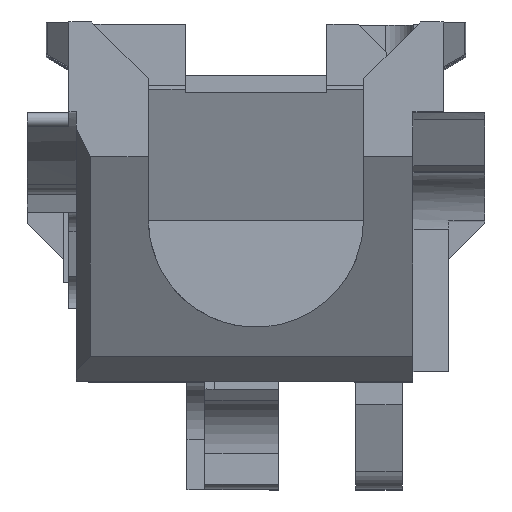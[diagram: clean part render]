
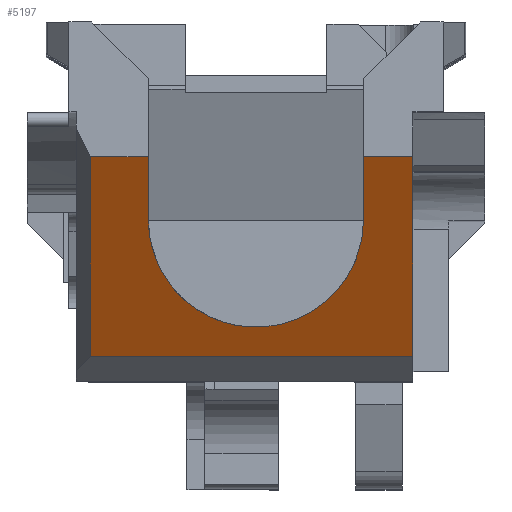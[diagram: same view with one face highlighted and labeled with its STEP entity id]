
A CAD part, top view. The second image highlights one B-rep face of the part: STEP entity #5197.
In plain terms, the highlighted planar face has unit normal (0, -0.5, 0.866).
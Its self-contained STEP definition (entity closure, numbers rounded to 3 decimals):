
#136=ELLIPSE('',#5634,6.928,6.);
#537=FACE_OUTER_BOUND('',#816,.T.);
#816=EDGE_LOOP('',(#4568,#4569,#4570,#4571,#4572,#4573,#4574,#4575));
#1097=LINE('',#7737,#1667);
#1274=LINE('',#8254,#1844);
#1280=LINE('',#8266,#1850);
#1281=LINE('',#8272,#1851);
#1358=LINE('',#8516,#1928);
#1398=LINE('',#8621,#1968);
#1400=LINE('',#8624,#1970);
#1667=VECTOR('',#6162,10.);
#1844=VECTOR('',#6629,10.);
#1850=VECTOR('',#6639,10.);
#1851=VECTOR('',#6646,10.);
#1928=VECTOR('',#6855,10.);
#1968=VECTOR('',#6979,10.);
#1970=VECTOR('',#6983,10.);
#2238=VERTEX_POINT('',#7734);
#2239=VERTEX_POINT('',#7736);
#2387=VERTEX_POINT('',#8251);
#2388=VERTEX_POINT('',#8253);
#2392=VERTEX_POINT('',#8264);
#2394=VERTEX_POINT('',#8271);
#2467=VERTEX_POINT('',#8515);
#2490=VERTEX_POINT('',#8619);
#2805=EDGE_CURVE('',#2238,#2239,#1097,.T.);
#3045=EDGE_CURVE('',#2387,#2388,#1274,.T.);
#3052=EDGE_CURVE('',#2387,#2392,#1280,.T.);
#3054=EDGE_CURVE('',#2394,#2239,#1281,.T.);
#3165=EDGE_CURVE('',#2467,#2388,#1358,.T.);
#3218=EDGE_CURVE('',#2490,#2238,#1398,.T.);
#3220=EDGE_CURVE('',#2467,#2490,#1400,.T.);
#3221=EDGE_CURVE('',#2392,#2394,#136,.T.);
#4568=ORIENTED_EDGE('',*,*,#3218,.F.);
#4569=ORIENTED_EDGE('',*,*,#3220,.F.);
#4570=ORIENTED_EDGE('',*,*,#3165,.T.);
#4571=ORIENTED_EDGE('',*,*,#3045,.F.);
#4572=ORIENTED_EDGE('',*,*,#3052,.T.);
#4573=ORIENTED_EDGE('',*,*,#3221,.T.);
#4574=ORIENTED_EDGE('',*,*,#3054,.T.);
#4575=ORIENTED_EDGE('',*,*,#2805,.F.);
#4963=PLANE('',#5633);
#5197=ADVANCED_FACE('',(#537),#4963,.F.);
#5633=AXIS2_PLACEMENT_3D('',#8623,#6981,#6982);
#5634=AXIS2_PLACEMENT_3D('',#8625,#6984,#6985);
#6162=DIRECTION('',(1.,0.,0.));
#6629=DIRECTION('',(1.,0.,0.));
#6639=DIRECTION('',(0.,-0.866,-0.5));
#6646=DIRECTION('',(0.,0.866,0.5));
#6855=DIRECTION('',(0.,0.866,0.5));
#6979=DIRECTION('',(0.,0.866,0.5));
#6981=DIRECTION('center_axis',(0.,0.5,-0.866));
#6982=DIRECTION('ref_axis',(0.,0.866,0.5));
#6983=DIRECTION('',(-1.,0.,0.));
#6984=DIRECTION('center_axis',(0.,0.5,-0.866));
#6985=DIRECTION('ref_axis',(0.,0.866,0.5));
#7734=CARTESIAN_POINT('',(-9.231,18.5,0.));
#7736=CARTESIAN_POINT('',(-6.,18.5,0.));
#7737=CARTESIAN_POINT('',(0.,18.5,0.));
#8251=CARTESIAN_POINT('',(6.,18.5,0.));
#8253=CARTESIAN_POINT('',(8.75,18.5,0.));
#8254=CARTESIAN_POINT('',(0.,18.5,0.));
#8264=CARTESIAN_POINT('',(6.,15.,-2.021));
#8266=CARTESIAN_POINT('',(6.,15.063,-1.985));
#8271=CARTESIAN_POINT('',(-6.,15.,-2.021));
#8272=CARTESIAN_POINT('',(-6.,10.938,-4.366));
#8515=CARTESIAN_POINT('',(8.75,7.375,-6.423));
#8516=CARTESIAN_POINT('',(8.75,-3.524,-12.715));
#8619=CARTESIAN_POINT('',(-9.231,7.375,-6.423));
#8621=CARTESIAN_POINT('',(-9.231,7.531,-6.333));
#8623=CARTESIAN_POINT('Origin',(0.,6.,-7.217));
#8624=CARTESIAN_POINT('',(0.,7.375,-6.423));
#8625=CARTESIAN_POINT('Origin',(0.,15.,-2.021));
